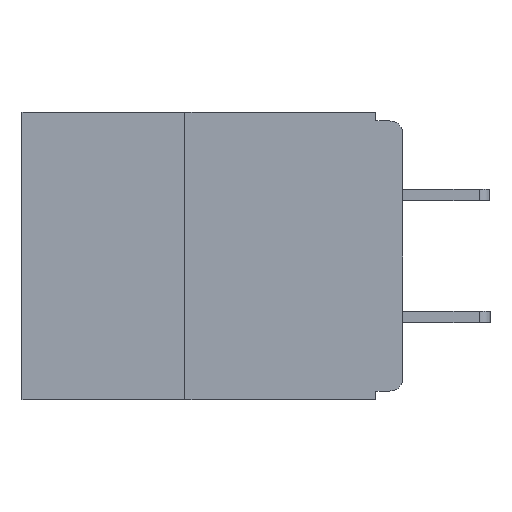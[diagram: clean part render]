
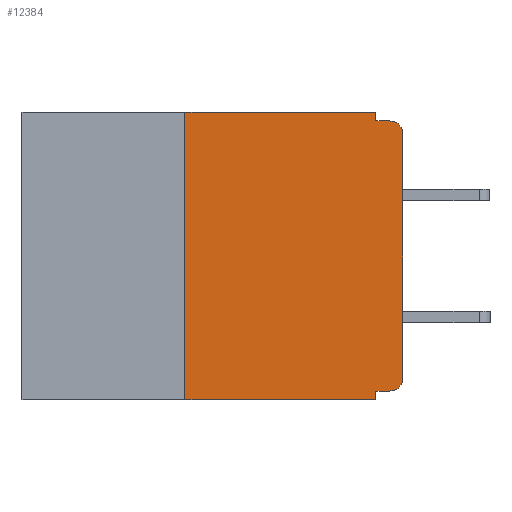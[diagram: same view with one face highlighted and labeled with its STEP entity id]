
A CAD part, left-side view. The second image highlights one B-rep face of the part: STEP entity #12384.
In plain terms, the highlighted planar face has unit normal (-1, 0, 0).
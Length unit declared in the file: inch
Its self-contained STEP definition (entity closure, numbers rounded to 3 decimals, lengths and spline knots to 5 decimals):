
#426 = DIRECTION ( 'NONE',  ( 0., -1., 0. ) ) ;
#1635 = EDGE_CURVE ( 'NONE', #20385, #13841, #21947, .T. ) ;
#2335 = CARTESIAN_POINT ( 'NONE',  ( 0., 0., -0.01 ) ) ;
#2405 = CARTESIAN_POINT ( 'NONE',  ( 0., 0.031, -0.01 ) ) ;
#2810 = CARTESIAN_POINT ( 'NONE',  ( 0., 0.031, -0.33 ) ) ;
#3014 = EDGE_CURVE ( 'NONE', #7254, #21380, #8771, .T. ) ;
#3055 = VERTEX_POINT ( 'NONE', #4406 ) ;
#3215 = CARTESIAN_POINT ( 'NONE',  ( 0., 0.015, -0.32 ) ) ;
#3315 = VECTOR ( 'NONE', #19108, 39.37008 ) ;
#3634 = CARTESIAN_POINT ( 'NONE',  ( 0., 0., -0.305 ) ) ;
#3775 = EDGE_CURVE ( 'NONE', #18619, #8087, #20923, .T. ) ;
#4406 = CARTESIAN_POINT ( 'NONE',  ( 0., 0.031, -0.33 ) ) ;
#4641 = ORIENTED_EDGE ( 'NONE', *, *, #22588, .F. ) ;
#4644 = PLANE ( 'NONE',  #19948 ) ;
#4818 = DIRECTION ( 'NONE',  ( 0., 1., 0. ) ) ;
#4868 = ORIENTED_EDGE ( 'NONE', *, *, #20843, .F. ) ;
#5210 = DIRECTION ( 'NONE',  ( 0., 0., -1. ) ) ;
#5298 = CARTESIAN_POINT ( 'NONE',  ( 0., 0.015, -0.025 ) ) ;
#5334 = DIRECTION ( 'NONE',  ( -1., 0., 0. ) ) ;
#5972 = VECTOR ( 'NONE', #8372, 39.37008 ) ;
#6497 = VERTEX_POINT ( 'NONE', #2405 ) ;
#6524 = DIRECTION ( 'NONE',  ( 1., 0., 0. ) ) ;
#7155 = ORIENTED_EDGE ( 'NONE', *, *, #7701, .F. ) ;
#7254 = VERTEX_POINT ( 'NONE', #15793 ) ;
#7701 = EDGE_CURVE ( 'NONE', #6497, #21380, #16961, .T. ) ;
#7717 = CARTESIAN_POINT ( 'NONE',  ( 0., 0.031, -0.32 ) ) ;
#7948 = CARTESIAN_POINT ( 'NONE',  ( 0., 0.031, 0. ) ) ;
#8087 = VERTEX_POINT ( 'NONE', #12700 ) ;
#8372 = DIRECTION ( 'NONE',  ( 0., 0., -1. ) ) ;
#8771 = CIRCLE ( 'NONE', #22522, 0.015 ) ;
#9435 = CARTESIAN_POINT ( 'NONE',  ( 0., 0.25, -0.33 ) ) ;
#9884 = EDGE_CURVE ( 'NONE', #22346, #18619, #17865, .T. ) ;
#9952 = LINE ( 'NONE', #21820, #14357 ) ;
#10153 = LINE ( 'NONE', #22603, #14557 ) ;
#10886 = LINE ( 'NONE', #2810, #5972 ) ;
#10952 = EDGE_CURVE ( 'NONE', #13841, #7254, #9952, .T. ) ;
#11014 = CARTESIAN_POINT ( 'NONE',  ( 0., 0.25, 0. ) ) ;
#11336 = DIRECTION ( 'NONE',  ( 0., 0., 1. ) ) ;
#11545 = DIRECTION ( 'NONE',  ( 0., -1., 0. ) ) ;
#12174 = VERTEX_POINT ( 'NONE', #7717 ) ;
#12384 = ADVANCED_FACE ( 'NONE', ( #19209 ), #4644, .F. ) ;
#12700 = CARTESIAN_POINT ( 'NONE',  ( 0., 0.031, 0. ) ) ;
#12998 = VECTOR ( 'NONE', #11336, 39.37008 ) ;
#13841 = VERTEX_POINT ( 'NONE', #3634 ) ;
#14010 = LINE ( 'NONE', #15880, #19505 ) ;
#14357 = VECTOR ( 'NONE', #21740, 39.37008 ) ;
#14557 = VECTOR ( 'NONE', #11545, 39.37008 ) ;
#14851 = ORIENTED_EDGE ( 'NONE', *, *, #9884, .F. ) ;
#15396 = VECTOR ( 'NONE', #17443, 39.37008 ) ;
#15654 = AXIS2_PLACEMENT_3D ( 'NONE', #20869, #16588, #16584 ) ;
#15674 = EDGE_LOOP ( 'NONE', ( #21036, #23894, #7155, #4641, #17996, #14851, #19856, #18215, #4868, #17048 ) ) ;
#15793 = CARTESIAN_POINT ( 'NONE',  ( 0., 0., -0.025 ) ) ;
#15880 = CARTESIAN_POINT ( 'NONE',  ( 0., 0., -0.32 ) ) ;
#16584 = DIRECTION ( 'NONE',  ( 0., 0., -1. ) ) ;
#16588 = DIRECTION ( 'NONE',  ( -1., 0., 0. ) ) ;
#16961 = LINE ( 'NONE', #2335, #21297 ) ;
#17048 = ORIENTED_EDGE ( 'NONE', *, *, #1635, .T. ) ;
#17443 = DIRECTION ( 'NONE',  ( 0., -1., 0. ) ) ;
#17519 = LINE ( 'NONE', #7948, #3315 ) ;
#17538 = CARTESIAN_POINT ( 'NONE',  ( 0., 0.437, 0. ) ) ;
#17557 = CARTESIAN_POINT ( 'NONE',  ( 0., 0.437, 0. ) ) ;
#17865 = LINE ( 'NONE', #9435, #12998 ) ;
#17996 = ORIENTED_EDGE ( 'NONE', *, *, #3775, .F. ) ;
#18215 = ORIENTED_EDGE ( 'NONE', *, *, #18972, .F. ) ;
#18619 = VERTEX_POINT ( 'NONE', #11014 ) ;
#18972 = EDGE_CURVE ( 'NONE', #12174, #3055, #10886, .T. ) ;
#19108 = DIRECTION ( 'NONE',  ( 0., 0., -1. ) ) ;
#19209 = FACE_OUTER_BOUND ( 'NONE', #15674, .T. ) ;
#19493 = DIRECTION ( 'NONE',  ( 0., 0., -1. ) ) ;
#19505 = VECTOR ( 'NONE', #4818, 39.37008 ) ;
#19856 = ORIENTED_EDGE ( 'NONE', *, *, #21253, .T. ) ;
#19948 = AXIS2_PLACEMENT_3D ( 'NONE', #17538, #6524, #19493 ) ;
#20314 = CARTESIAN_POINT ( 'NONE',  ( 0., 0.25, -0.33 ) ) ;
#20385 = VERTEX_POINT ( 'NONE', #3215 ) ;
#20843 = EDGE_CURVE ( 'NONE', #20385, #12174, #14010, .T. ) ;
#20869 = CARTESIAN_POINT ( 'NONE',  ( 0., 0.015, -0.305 ) ) ;
#20923 = LINE ( 'NONE', #17557, #15396 ) ;
#21036 = ORIENTED_EDGE ( 'NONE', *, *, #10952, .T. ) ;
#21253 = EDGE_CURVE ( 'NONE', #22346, #3055, #10153, .T. ) ;
#21297 = VECTOR ( 'NONE', #426, 39.37008 ) ;
#21380 = VERTEX_POINT ( 'NONE', #22908 ) ;
#21740 = DIRECTION ( 'NONE',  ( 0., 0., 1. ) ) ;
#21820 = CARTESIAN_POINT ( 'NONE',  ( 0., 0., 0. ) ) ;
#21947 = CIRCLE ( 'NONE', #15654, 0.015 ) ;
#22346 = VERTEX_POINT ( 'NONE', #20314 ) ;
#22522 = AXIS2_PLACEMENT_3D ( 'NONE', #5298, #5334, #5210 ) ;
#22588 = EDGE_CURVE ( 'NONE', #8087, #6497, #17519, .T. ) ;
#22603 = CARTESIAN_POINT ( 'NONE',  ( 0., 0.437, -0.33 ) ) ;
#22908 = CARTESIAN_POINT ( 'NONE',  ( 0., 0.015, -0.01 ) ) ;
#23894 = ORIENTED_EDGE ( 'NONE', *, *, #3014, .T. ) ;
